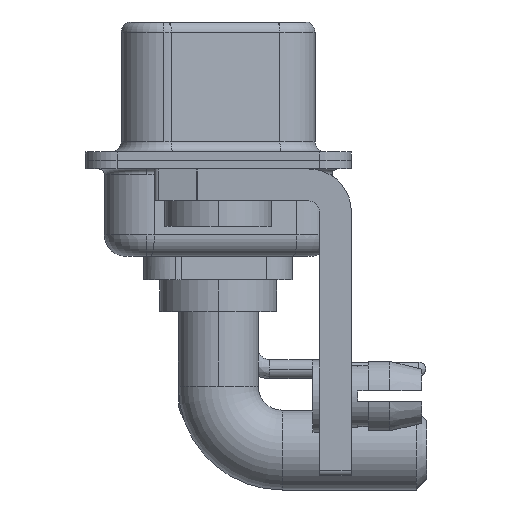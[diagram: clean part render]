
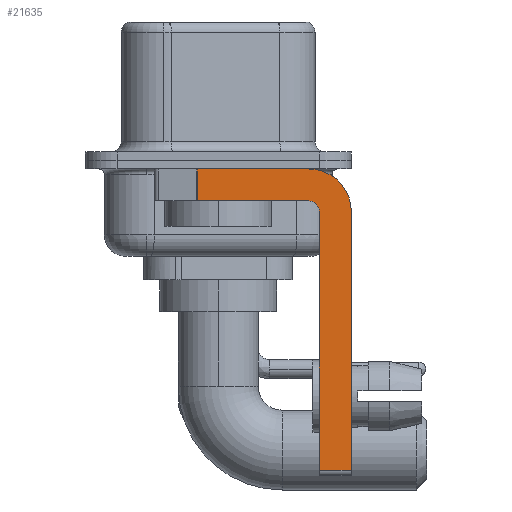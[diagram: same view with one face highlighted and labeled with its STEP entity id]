
A CAD part, left-side view. The second image highlights one B-rep face of the part: STEP entity #21635.
In plain terms, the highlighted planar face has unit normal (-1, 0, 0).
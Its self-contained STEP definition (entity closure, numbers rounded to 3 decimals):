
#370 = ORIENTED_EDGE ( 'NONE', *, *, #23366, .F. ) ;
#416 = AXIS2_PLACEMENT_3D ( 'NONE', #13937, #18274, #25799 ) ;
#569 = CARTESIAN_POINT ( 'NONE',  ( -2.9, -4.25, -2.4 ) ) ;
#1035 = DIRECTION ( 'NONE',  ( 0., -1., 0. ) ) ;
#1388 = VERTEX_POINT ( 'NONE', #8785 ) ;
#2800 = CARTESIAN_POINT ( 'NONE',  ( -2.9, 0.978, -1.9 ) ) ;
#3830 = EDGE_CURVE ( 'NONE', #13485, #22400, #29797, .T. ) ;
#4367 = AXIS2_PLACEMENT_3D ( 'NONE', #7742, #7439, #26225 ) ;
#5548 = VERTEX_POINT ( 'NONE', #29125 ) ;
#5557 = CARTESIAN_POINT ( 'NONE',  ( -2.9, 0.978, -0.4 ) ) ;
#5880 = LINE ( 'NONE', #23077, #21615 ) ;
#6895 = VERTEX_POINT ( 'NONE', #5557 ) ;
#7218 = DIRECTION ( 'NONE',  ( 0., 0., -1. ) ) ;
#7410 = EDGE_CURVE ( 'NONE', #19765, #5548, #8746, .T. ) ;
#7439 = DIRECTION ( 'NONE',  ( -1., 0., 0. ) ) ;
#7742 = CARTESIAN_POINT ( 'NONE',  ( -2.9, -4.25, -2.4 ) ) ;
#7864 = VECTOR ( 'NONE', #8269, 1000. ) ;
#8269 = DIRECTION ( 'NONE',  ( 0., 0., -1. ) ) ;
#8671 = DIRECTION ( 'NONE',  ( 0., 1., 0. ) ) ;
#8729 = ORIENTED_EDGE ( 'NONE', *, *, #7410, .T. ) ;
#8746 = LINE ( 'NONE', #17536, #16575 ) ;
#8785 = CARTESIAN_POINT ( 'NONE',  ( -2.9, -4.25, -0.4 ) ) ;
#8899 = EDGE_CURVE ( 'NONE', #22536, #13485, #13706, .T. ) ;
#10269 = LINE ( 'NONE', #19977, #7864 ) ;
#11375 = DIRECTION ( 'NONE',  ( 0., 0., -1. ) ) ;
#11434 = CARTESIAN_POINT ( 'NONE',  ( -2.9, -4.25, -1.9 ) ) ;
#11678 = PLANE ( 'NONE',  #13685 ) ;
#11843 = EDGE_CURVE ( 'NONE', #1388, #26754, #22582, .T. ) ;
#12561 = LINE ( 'NONE', #24732, #13249 ) ;
#13249 = VECTOR ( 'NONE', #22425, 1000. ) ;
#13485 = VERTEX_POINT ( 'NONE', #24585 ) ;
#13685 = AXIS2_PLACEMENT_3D ( 'NONE', #569, #28331, #7218 ) ;
#13706 = CIRCLE ( 'NONE', #4367, 0.5 ) ;
#13937 = CARTESIAN_POINT ( 'NONE',  ( -2.9, -4.25, -2.4 ) ) ;
#14090 = EDGE_CURVE ( 'NONE', #6895, #1388, #12561, .T. ) ;
#15481 = EDGE_CURVE ( 'NONE', #19765, #22536, #26327, .T. ) ;
#16575 = VECTOR ( 'NONE', #1035, 1000. ) ;
#17398 = CARTESIAN_POINT ( 'NONE',  ( -2.9, -4.75, -14.8 ) ) ;
#17536 = CARTESIAN_POINT ( 'NONE',  ( -2.9, -4.25, -14.55 ) ) ;
#17667 = ORIENTED_EDGE ( 'NONE', *, *, #23682, .T. ) ;
#18274 = DIRECTION ( 'NONE',  ( 1., 0., 0. ) ) ;
#18284 = CARTESIAN_POINT ( 'NONE',  ( -2.9, -4.75, -2.4 ) ) ;
#18381 = ORIENTED_EDGE ( 'NONE', *, *, #15481, .F. ) ;
#18436 = ORIENTED_EDGE ( 'NONE', *, *, #11843, .F. ) ;
#19165 = CARTESIAN_POINT ( 'NONE',  ( -2.9, -6.25, -2.4 ) ) ;
#19765 = VERTEX_POINT ( 'NONE', #24986 ) ;
#19977 = CARTESIAN_POINT ( 'NONE',  ( -2.9, 0.978, -1.9 ) ) ;
#21615 = VECTOR ( 'NONE', #11375, 1000. ) ;
#21635 = ADVANCED_FACE ( 'NONE', ( #26007 ), #11678, .F. ) ;
#22244 = VECTOR ( 'NONE', #8671, 1000. ) ;
#22400 = VERTEX_POINT ( 'NONE', #2800 ) ;
#22425 = DIRECTION ( 'NONE',  ( 0., -1., 0. ) ) ;
#22536 = VERTEX_POINT ( 'NONE', #18284 ) ;
#22582 = CIRCLE ( 'NONE', #416, 2. ) ;
#23077 = CARTESIAN_POINT ( 'NONE',  ( -2.9, -6.25, -2.4 ) ) ;
#23366 = EDGE_CURVE ( 'NONE', #26754, #5548, #5880, .T. ) ;
#23682 = EDGE_CURVE ( 'NONE', #6895, #22400, #10269, .T. ) ;
#24320 = DIRECTION ( 'NONE',  ( 0., 0., 1. ) ) ;
#24441 = VECTOR ( 'NONE', #24320, 1000. ) ;
#24585 = CARTESIAN_POINT ( 'NONE',  ( -2.9, -4.25, -1.9 ) ) ;
#24593 = ORIENTED_EDGE ( 'NONE', *, *, #8899, .F. ) ;
#24732 = CARTESIAN_POINT ( 'NONE',  ( -2.9, 3., -0.4 ) ) ;
#24986 = CARTESIAN_POINT ( 'NONE',  ( -2.9, -4.75, -14.55 ) ) ;
#25799 = DIRECTION ( 'NONE',  ( 0., 0., -1. ) ) ;
#26007 = FACE_OUTER_BOUND ( 'NONE', #26353, .T. ) ;
#26225 = DIRECTION ( 'NONE',  ( 0., 0., 1. ) ) ;
#26327 = LINE ( 'NONE', #17398, #24441 ) ;
#26353 = EDGE_LOOP ( 'NONE', ( #27626, #17667, #30157, #24593, #18381, #8729, #370, #18436 ) ) ;
#26754 = VERTEX_POINT ( 'NONE', #19165 ) ;
#27626 = ORIENTED_EDGE ( 'NONE', *, *, #14090, .F. ) ;
#28331 = DIRECTION ( 'NONE',  ( 1., 0., 0. ) ) ;
#29125 = CARTESIAN_POINT ( 'NONE',  ( -2.9, -6.25, -14.55 ) ) ;
#29797 = LINE ( 'NONE', #11434, #22244 ) ;
#30157 = ORIENTED_EDGE ( 'NONE', *, *, #3830, .F. ) ;
